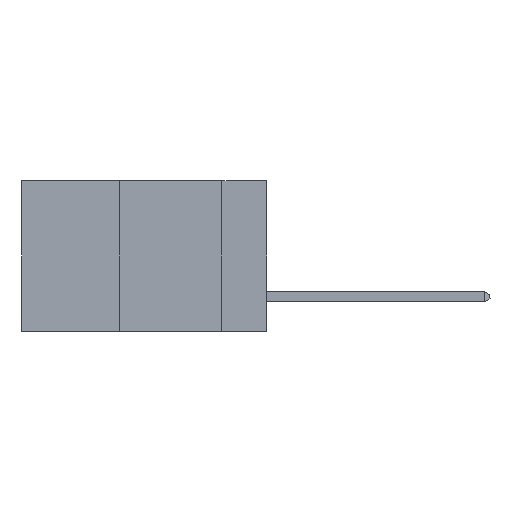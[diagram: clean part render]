
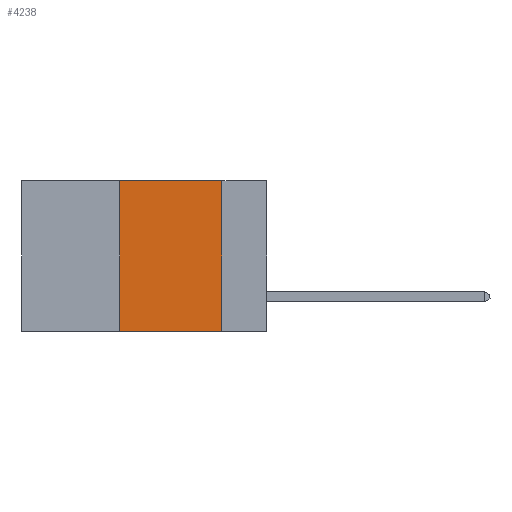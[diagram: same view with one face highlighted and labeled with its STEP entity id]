
A CAD part, left-side view. The second image highlights one B-rep face of the part: STEP entity #4238.
In plain terms, the highlighted planar face has unit normal (-1, 0, 0).
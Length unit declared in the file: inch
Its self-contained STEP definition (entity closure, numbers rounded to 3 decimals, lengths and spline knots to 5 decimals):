
#246 = CARTESIAN_POINT ( 'NONE',  ( 0., 0.6, 0. ) ) ;
#1637 = LINE ( 'NONE', #10099, #6314 ) ;
#1727 = ORIENTED_EDGE ( 'NONE', *, *, #7513, .T. ) ;
#1745 = DIRECTION ( 'NONE',  ( 0., -1., 0. ) ) ;
#1787 = DIRECTION ( 'NONE',  ( 0., 0., 1. ) ) ;
#1933 = AXIS2_PLACEMENT_3D ( 'NONE', #8794, #3540, #9248 ) ;
#2908 = DIRECTION ( 'NONE',  ( 0., 0., -1. ) ) ;
#3190 = LINE ( 'NONE', #13743, #11744 ) ;
#3540 = DIRECTION ( 'NONE',  ( 1., 0., 0. ) ) ;
#4039 = VERTEX_POINT ( 'NONE', #4203 ) ;
#4203 = CARTESIAN_POINT ( 'NONE',  ( 0., 0.11, 0. ) ) ;
#4238 = ADVANCED_FACE ( 'NONE', ( #17333 ), #10051, .F. ) ;
#4752 = VECTOR ( 'NONE', #1745, 39.37008 ) ;
#5882 = LINE ( 'NONE', #9037, #12526 ) ;
#5892 = VERTEX_POINT ( 'NONE', #13873 ) ;
#6314 = VECTOR ( 'NONE', #1787, 39.37008 ) ;
#6627 = EDGE_CURVE ( 'NONE', #7995, #5892, #1637, .T. ) ;
#7190 = EDGE_CURVE ( 'NONE', #4039, #11156, #3190, .T. ) ;
#7513 = EDGE_CURVE ( 'NONE', #7995, #11156, #5882, .T. ) ;
#7995 = VERTEX_POINT ( 'NONE', #10126 ) ;
#8794 = CARTESIAN_POINT ( 'NONE',  ( 0., 0.6, 0. ) ) ;
#9037 = CARTESIAN_POINT ( 'NONE',  ( 0., 0.6, -0.37 ) ) ;
#9248 = DIRECTION ( 'NONE',  ( 0., 0., -1. ) ) ;
#9448 = ORIENTED_EDGE ( 'NONE', *, *, #7190, .F. ) ;
#10051 = PLANE ( 'NONE',  #1933 ) ;
#10099 = CARTESIAN_POINT ( 'NONE',  ( 0., 0.36, 0. ) ) ;
#10126 = CARTESIAN_POINT ( 'NONE',  ( 0., 0.36, -0.37 ) ) ;
#10424 = DIRECTION ( 'NONE',  ( 0., -1., 0. ) ) ;
#11156 = VERTEX_POINT ( 'NONE', #13630 ) ;
#11713 = EDGE_LOOP ( 'NONE', ( #9448, #13624, #14812, #1727 ) ) ;
#11744 = VECTOR ( 'NONE', #2908, 39.37008 ) ;
#11947 = LINE ( 'NONE', #246, #4752 ) ;
#12526 = VECTOR ( 'NONE', #10424, 39.37008 ) ;
#13624 = ORIENTED_EDGE ( 'NONE', *, *, #15052, .F. ) ;
#13630 = CARTESIAN_POINT ( 'NONE',  ( 0., 0.11, -0.37 ) ) ;
#13743 = CARTESIAN_POINT ( 'NONE',  ( 0., 0.11, 0. ) ) ;
#13873 = CARTESIAN_POINT ( 'NONE',  ( 0., 0.36, 0. ) ) ;
#14812 = ORIENTED_EDGE ( 'NONE', *, *, #6627, .F. ) ;
#15052 = EDGE_CURVE ( 'NONE', #5892, #4039, #11947, .T. ) ;
#17333 = FACE_OUTER_BOUND ( 'NONE', #11713, .T. ) ;
